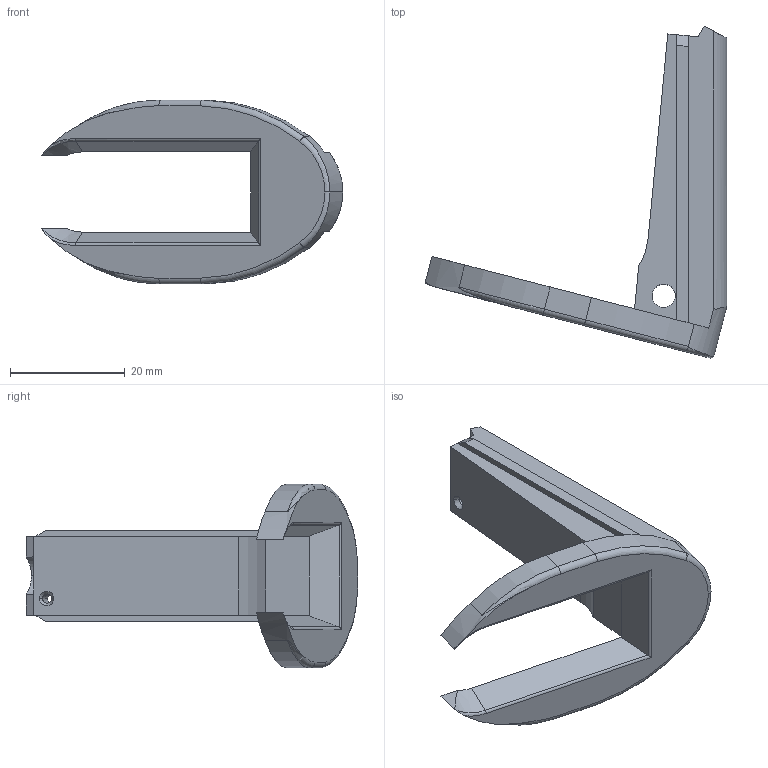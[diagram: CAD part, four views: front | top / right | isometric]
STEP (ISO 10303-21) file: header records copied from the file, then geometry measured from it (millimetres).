
FILE_DESCRIPTION (( 'STEP AP214' ), '1' );
FILE_NAME ('5503841.STEP', '2013-07-30T15:11:23', ( 'Asher' ), ( '' ), 'SwSTEP 2.0', 'SolidWorks 2013', '' );
FILE_SCHEMA (( 'AUTOMOTIVE_DESIGN' ));
Length unit declared in the file: millimetre
Products named in the file (1): 5503841
Bounding box: 52.56 x 57.85 x 32.03 mm (x, y, z)
Volume: 10463.1 mm3; surface area: 6334.4 mm2
Topology: 1 solids, 1 shells, 67 faces, 182 edges, 115 vertices
Faces by surface type: plane 30, cylinder 21, torus 10, cone 6
Entity records: 2344 total; most frequent: CARTESIAN_POINT 663, ORIENTED_EDGE 360, DIRECTION 327, EDGE_CURVE 180, AXIS2_PLACEMENT_3D 115, VERTEX_POINT 115, LINE 97, VECTOR 97
